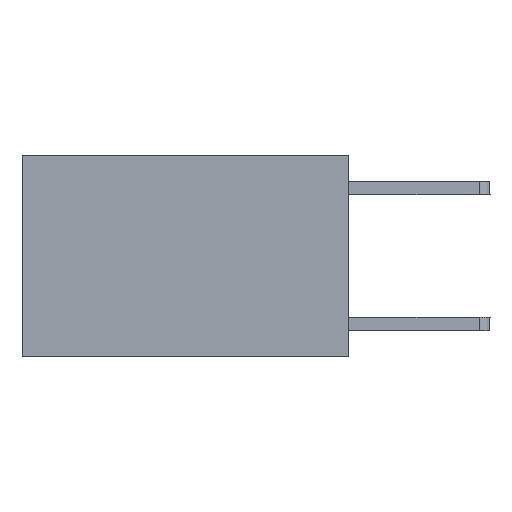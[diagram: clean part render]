
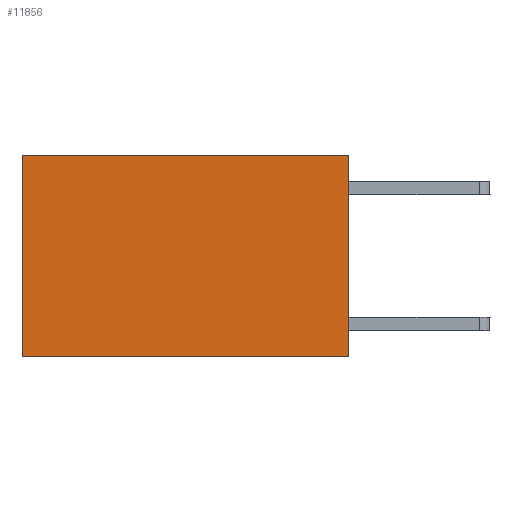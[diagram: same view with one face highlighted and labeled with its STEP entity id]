
A CAD part, left-side view. The second image highlights one B-rep face of the part: STEP entity #11856.
In plain terms, the highlighted planar face has unit normal (-1, 0, 0).
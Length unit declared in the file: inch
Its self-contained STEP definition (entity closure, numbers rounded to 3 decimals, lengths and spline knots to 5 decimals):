
#83 = LINE ( 'NONE', #3681, #11062 ) ;
#265 = CARTESIAN_POINT ( 'NONE',  ( 0.2625, 0., 0. ) ) ;
#322 = DIRECTION ( 'NONE',  ( 0., 0., -1. ) ) ;
#497 = ORIENTED_EDGE ( 'NONE', *, *, #5835, .T. ) ;
#747 = DIRECTION ( 'NONE',  ( 0., 0., -1. ) ) ;
#1121 = VERTEX_POINT ( 'NONE', #10034 ) ;
#1200 = ORIENTED_EDGE ( 'NONE', *, *, #2150, .F. ) ;
#1415 = ORIENTED_EDGE ( 'NONE', *, *, #3388, .T. ) ;
#1636 = CARTESIAN_POINT ( 'NONE',  ( 0.2625, 0., 0. ) ) ;
#1843 = DIRECTION ( 'NONE',  ( 0., 1., 0. ) ) ;
#2150 = EDGE_CURVE ( 'NONE', #3335, #8008, #83, .T. ) ;
#2566 = EDGE_LOOP ( 'NONE', ( #1415, #1200, #7104, #497 ) ) ;
#3335 = VERTEX_POINT ( 'NONE', #9394 ) ;
#3388 = EDGE_CURVE ( 'NONE', #1121, #8008, #4071, .T. ) ;
#3681 = CARTESIAN_POINT ( 'NONE',  ( 0.2625, 0., -0.37 ) ) ;
#4037 = CARTESIAN_POINT ( 'NONE',  ( 0.2625, 0., 0. ) ) ;
#4071 = LINE ( 'NONE', #6916, #6674 ) ;
#4189 = CARTESIAN_POINT ( 'NONE',  ( 0.2625, 0.6, -0.37 ) ) ;
#4339 = DIRECTION ( 'NONE',  ( 0., 0., -1. ) ) ;
#5824 = LINE ( 'NONE', #265, #10973 ) ;
#5835 = EDGE_CURVE ( 'NONE', #11918, #1121, #5824, .T. ) ;
#6258 = DIRECTION ( 'NONE',  ( 0., 1., 0. ) ) ;
#6315 = LINE ( 'NONE', #1636, #10740 ) ;
#6674 = VECTOR ( 'NONE', #4339, 39.37008 ) ;
#6916 = CARTESIAN_POINT ( 'NONE',  ( 0.2625, 0.6, 0. ) ) ;
#7104 = ORIENTED_EDGE ( 'NONE', *, *, #8283, .F. ) ;
#7656 = PLANE ( 'NONE',  #8982 ) ;
#8008 = VERTEX_POINT ( 'NONE', #4189 ) ;
#8283 = EDGE_CURVE ( 'NONE', #11918, #3335, #6315, .T. ) ;
#8982 = AXIS2_PLACEMENT_3D ( 'NONE', #4037, #10400, #322 ) ;
#9394 = CARTESIAN_POINT ( 'NONE',  ( 0.2625, 0., -0.37 ) ) ;
#9594 = FACE_OUTER_BOUND ( 'NONE', #2566, .T. ) ;
#10034 = CARTESIAN_POINT ( 'NONE',  ( 0.2625, 0.6, 0. ) ) ;
#10400 = DIRECTION ( 'NONE',  ( 1., 0., 0. ) ) ;
#10520 = CARTESIAN_POINT ( 'NONE',  ( 0.2625, 0., 0. ) ) ;
#10740 = VECTOR ( 'NONE', #747, 39.37008 ) ;
#10973 = VECTOR ( 'NONE', #6258, 39.37008 ) ;
#11062 = VECTOR ( 'NONE', #1843, 39.37008 ) ;
#11856 = ADVANCED_FACE ( 'NONE', ( #9594 ), #7656, .F. ) ;
#11918 = VERTEX_POINT ( 'NONE', #10520 ) ;
